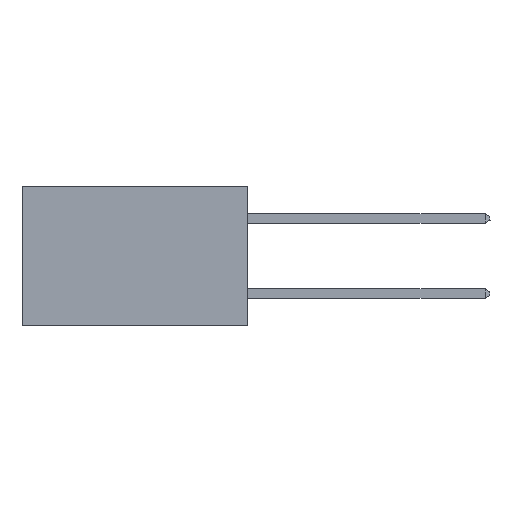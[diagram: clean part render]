
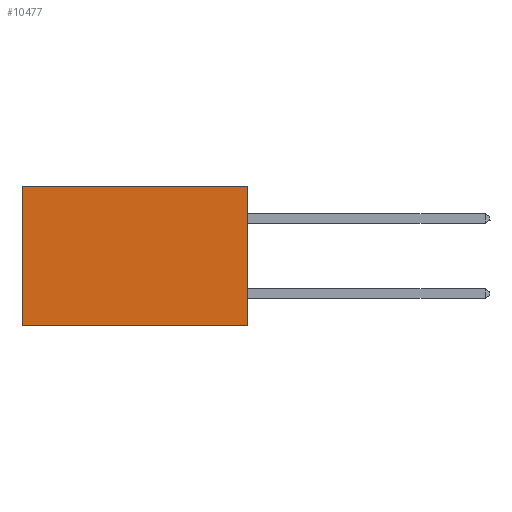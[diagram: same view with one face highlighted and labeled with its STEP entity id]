
A CAD part, left-side view. The second image highlights one B-rep face of the part: STEP entity #10477.
In plain terms, the highlighted planar face has unit normal (-1, 0, 0).
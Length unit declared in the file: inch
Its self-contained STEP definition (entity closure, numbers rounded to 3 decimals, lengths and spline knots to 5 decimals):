
#48 = FACE_OUTER_BOUND ( 'NONE', #16160, .T. ) ;
#190 = DIRECTION ( 'NONE',  ( 0., 0., -1. ) ) ;
#216 = ORIENTED_EDGE ( 'NONE', *, *, #19531, .F. ) ;
#726 = VERTEX_POINT ( 'NONE', #20048 ) ;
#764 = ORIENTED_EDGE ( 'NONE', *, *, #11761, .T. ) ;
#892 = EDGE_CURVE ( 'NONE', #726, #17141, #5151, .T. ) ;
#1297 = CARTESIAN_POINT ( 'NONE',  ( 0.2615, 0., -0.37 ) ) ;
#1378 = DIRECTION ( 'NONE',  ( 1., 0., 0. ) ) ;
#1839 = VECTOR ( 'NONE', #10736, 39.37008 ) ;
#3335 = VERTEX_POINT ( 'NONE', #20087 ) ;
#5151 = LINE ( 'NONE', #16037, #10944 ) ;
#6640 = LINE ( 'NONE', #17635, #1839 ) ;
#6679 = CARTESIAN_POINT ( 'NONE',  ( 0.2615, 0.6, 0. ) ) ;
#7885 = VECTOR ( 'NONE', #190, 39.37008 ) ;
#7918 = DIRECTION ( 'NONE',  ( 0., 1., 0. ) ) ;
#8509 = VERTEX_POINT ( 'NONE', #12166 ) ;
#9392 = EDGE_CURVE ( 'NONE', #8509, #3335, #6640, .T. ) ;
#10403 = AXIS2_PLACEMENT_3D ( 'NONE', #1297, #1378, #13772 ) ;
#10477 = ADVANCED_FACE ( 'NONE', ( #48 ), #17158, .F. ) ;
#10736 = DIRECTION ( 'NONE',  ( 0., 1., 0. ) ) ;
#10944 = VECTOR ( 'NONE', #7918, 39.37008 ) ;
#11761 = EDGE_CURVE ( 'NONE', #17141, #3335, #18207, .T. ) ;
#12166 = CARTESIAN_POINT ( 'NONE',  ( 0.2615, 0., -0.37 ) ) ;
#12677 = CARTESIAN_POINT ( 'NONE',  ( 0.2615, 0., -0.37 ) ) ;
#13772 = DIRECTION ( 'NONE',  ( 0., 0., -1. ) ) ;
#16037 = CARTESIAN_POINT ( 'NONE',  ( 0.2615, 0., 0. ) ) ;
#16160 = EDGE_LOOP ( 'NONE', ( #764, #21216, #216, #17370 ) ) ;
#17036 = CARTESIAN_POINT ( 'NONE',  ( 0.2615, 0.6, -0.37 ) ) ;
#17133 = LINE ( 'NONE', #12677, #7885 ) ;
#17141 = VERTEX_POINT ( 'NONE', #6679 ) ;
#17158 = PLANE ( 'NONE',  #10403 ) ;
#17370 = ORIENTED_EDGE ( 'NONE', *, *, #892, .T. ) ;
#17635 = CARTESIAN_POINT ( 'NONE',  ( 0.2615, 0., -0.37 ) ) ;
#18207 = LINE ( 'NONE', #17036, #22181 ) ;
#18743 = DIRECTION ( 'NONE',  ( 0., 0., -1. ) ) ;
#19531 = EDGE_CURVE ( 'NONE', #726, #8509, #17133, .T. ) ;
#20048 = CARTESIAN_POINT ( 'NONE',  ( 0.2615, 0., 0. ) ) ;
#20087 = CARTESIAN_POINT ( 'NONE',  ( 0.2615, 0.6, -0.37 ) ) ;
#21216 = ORIENTED_EDGE ( 'NONE', *, *, #9392, .F. ) ;
#22181 = VECTOR ( 'NONE', #18743, 39.37008 ) ;
